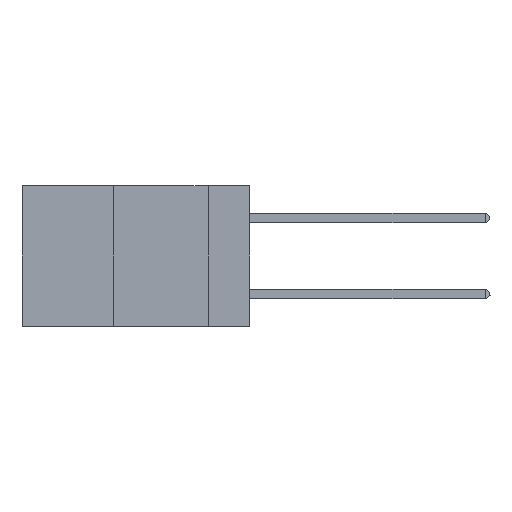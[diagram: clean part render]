
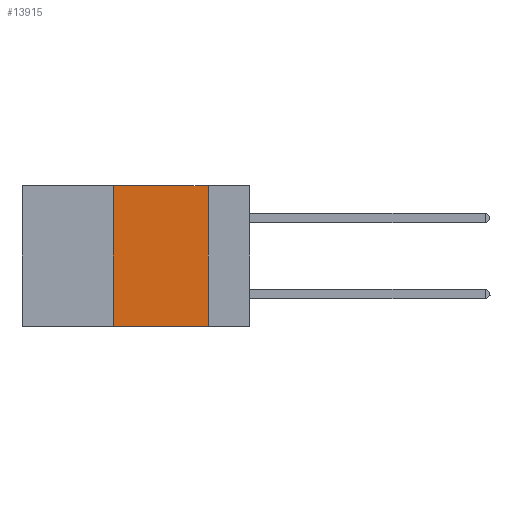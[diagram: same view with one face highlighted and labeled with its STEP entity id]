
A CAD part, left-side view. The second image highlights one B-rep face of the part: STEP entity #13915.
In plain terms, the highlighted planar face has unit normal (-1, 0, 0).
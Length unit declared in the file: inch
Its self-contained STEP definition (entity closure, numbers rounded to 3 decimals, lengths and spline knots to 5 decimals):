
#110 = VERTEX_POINT ( 'NONE', #12891 ) ;
#381 = DIRECTION ( 'NONE',  ( 0., 0., 1. ) ) ;
#448 = VECTOR ( 'NONE', #5448, 39.37008 ) ;
#472 = EDGE_LOOP ( 'NONE', ( #10886, #12095, #8833, #8823 ) ) ;
#664 = AXIS2_PLACEMENT_3D ( 'NONE', #2955, #17482, #5995 ) ;
#905 = LINE ( 'NONE', #16921, #448 ) ;
#956 = VECTOR ( 'NONE', #381, 39.37008 ) ;
#1243 = CARTESIAN_POINT ( 'NONE',  ( 0., 0.36, -0.37 ) ) ;
#1462 = VERTEX_POINT ( 'NONE', #10694 ) ;
#2955 = CARTESIAN_POINT ( 'NONE',  ( 0., 0.6, 0. ) ) ;
#3129 = VERTEX_POINT ( 'NONE', #1243 ) ;
#4929 = VERTEX_POINT ( 'NONE', #14042 ) ;
#5448 = DIRECTION ( 'NONE',  ( 0., -1., 0. ) ) ;
#5995 = DIRECTION ( 'NONE',  ( 0., 0., -1. ) ) ;
#6275 = LINE ( 'NONE', #7640, #11728 ) ;
#7640 = CARTESIAN_POINT ( 'NONE',  ( 0., 0.6, -0.37 ) ) ;
#8823 = ORIENTED_EDGE ( 'NONE', *, *, #14784, .T. ) ;
#8833 = ORIENTED_EDGE ( 'NONE', *, *, #14761, .F. ) ;
#10240 = PLANE ( 'NONE',  #664 ) ;
#10574 = VECTOR ( 'NONE', #14590, 39.37008 ) ;
#10694 = CARTESIAN_POINT ( 'NONE',  ( 0., 0.11, -0.37 ) ) ;
#10886 = ORIENTED_EDGE ( 'NONE', *, *, #18261, .F. ) ;
#11724 = LINE ( 'NONE', #13156, #10574 ) ;
#11728 = VECTOR ( 'NONE', #13458, 39.37008 ) ;
#12095 = ORIENTED_EDGE ( 'NONE', *, *, #16241, .F. ) ;
#12891 = CARTESIAN_POINT ( 'NONE',  ( 0., 0.36, 0. ) ) ;
#13156 = CARTESIAN_POINT ( 'NONE',  ( 0., 0.11, 0. ) ) ;
#13230 = FACE_OUTER_BOUND ( 'NONE', #472, .T. ) ;
#13458 = DIRECTION ( 'NONE',  ( 0., -1., 0. ) ) ;
#13915 = ADVANCED_FACE ( 'NONE', ( #13230 ), #10240, .F. ) ;
#14042 = CARTESIAN_POINT ( 'NONE',  ( 0., 0.11, 0. ) ) ;
#14590 = DIRECTION ( 'NONE',  ( 0., 0., -1. ) ) ;
#14761 = EDGE_CURVE ( 'NONE', #3129, #110, #17241, .T. ) ;
#14784 = EDGE_CURVE ( 'NONE', #3129, #1462, #6275, .T. ) ;
#16241 = EDGE_CURVE ( 'NONE', #110, #4929, #905, .T. ) ;
#16921 = CARTESIAN_POINT ( 'NONE',  ( 0., 0.6, 0. ) ) ;
#17241 = LINE ( 'NONE', #17636, #956 ) ;
#17482 = DIRECTION ( 'NONE',  ( 1., 0., 0. ) ) ;
#17636 = CARTESIAN_POINT ( 'NONE',  ( 0., 0.36, 0. ) ) ;
#18261 = EDGE_CURVE ( 'NONE', #4929, #1462, #11724, .T. ) ;
